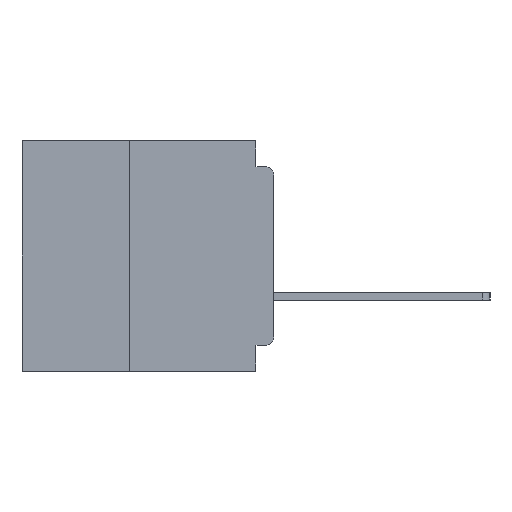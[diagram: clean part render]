
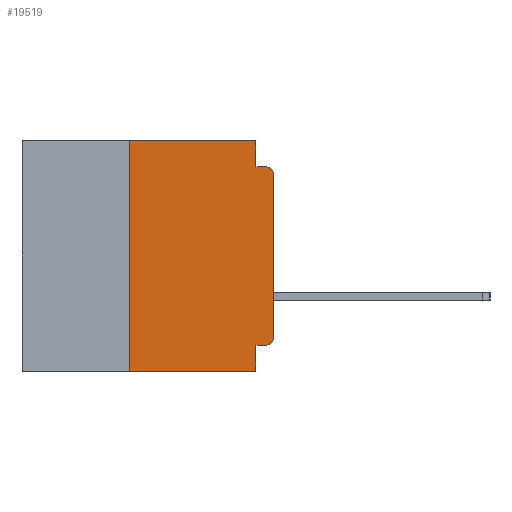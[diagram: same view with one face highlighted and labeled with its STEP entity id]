
A CAD part, left-side view. The second image highlights one B-rep face of the part: STEP entity #19519.
In plain terms, the highlighted planar face has unit normal (-1, 0, 0).
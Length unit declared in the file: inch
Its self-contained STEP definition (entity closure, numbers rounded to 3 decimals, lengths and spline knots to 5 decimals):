
#126 = ORIENTED_EDGE ( 'NONE', *, *, #12159, .T. ) ;
#327 = ORIENTED_EDGE ( 'NONE', *, *, #18618, .T. ) ;
#857 = ORIENTED_EDGE ( 'NONE', *, *, #13022, .F. ) ;
#1304 = ORIENTED_EDGE ( 'NONE', *, *, #26795, .F. ) ;
#1776 = LINE ( 'NONE', #21412, #37938 ) ;
#1802 = AXIS2_PLACEMENT_3D ( 'NONE', #40153, #40103, #40090 ) ;
#2200 = LINE ( 'NONE', #25122, #36204 ) ;
#2381 = CARTESIAN_POINT ( 'NONE',  ( 0., 0.25, -0.4 ) ) ;
#2428 = EDGE_CURVE ( 'NONE', #28921, #13755, #2200, .T. ) ;
#3907 = ORIENTED_EDGE ( 'NONE', *, *, #2428, .F. ) ;
#3928 = DIRECTION ( 'NONE',  ( 0., 0., 1. ) ) ;
#4588 = LINE ( 'NONE', #12384, #31452 ) ;
#4768 = CARTESIAN_POINT ( 'NONE',  ( 0., 0.437, 0. ) ) ;
#5545 = LINE ( 'NONE', #24265, #41652 ) ;
#5614 = VERTEX_POINT ( 'NONE', #10457 ) ;
#5684 = DIRECTION ( 'NONE',  ( 0., 1., 0. ) ) ;
#6616 = CARTESIAN_POINT ( 'NONE',  ( 0., 0.015, -0.045 ) ) ;
#6877 = EDGE_CURVE ( 'NONE', #5614, #39011, #18066, .T. ) ;
#7817 = ORIENTED_EDGE ( 'NONE', *, *, #22107, .F. ) ;
#8305 = DIRECTION ( 'NONE',  ( 0., 0., -1. ) ) ;
#8378 = ORIENTED_EDGE ( 'NONE', *, *, #15038, .T. ) ;
#8770 = CARTESIAN_POINT ( 'NONE',  ( 0., 0., -0.045 ) ) ;
#8804 = VECTOR ( 'NONE', #36818, 39.37008 ) ;
#10457 = CARTESIAN_POINT ( 'NONE',  ( 0., 0.015, -0.355 ) ) ;
#10784 = ORIENTED_EDGE ( 'NONE', *, *, #12684, .F. ) ;
#10994 = ORIENTED_EDGE ( 'NONE', *, *, #32732, .F. ) ;
#12159 = EDGE_CURVE ( 'NONE', #39011, #40071, #1776, .T. ) ;
#12169 = ORIENTED_EDGE ( 'NONE', *, *, #6877, .T. ) ;
#12384 = CARTESIAN_POINT ( 'NONE',  ( 0., 0.031, 0. ) ) ;
#12684 = EDGE_CURVE ( 'NONE', #27135, #31241, #5545, .T. ) ;
#13022 = EDGE_CURVE ( 'NONE', #45213, #23433, #44838, .T. ) ;
#13112 = CARTESIAN_POINT ( 'NONE',  ( 0., 0.437, -0.4 ) ) ;
#13446 = LINE ( 'NONE', #44415, #22800 ) ;
#13755 = VERTEX_POINT ( 'NONE', #16778 ) ;
#15038 = EDGE_CURVE ( 'NONE', #40482, #31241, #15154, .T. ) ;
#15154 = LINE ( 'NONE', #13112, #32748 ) ;
#16163 = EDGE_LOOP ( 'NONE', ( #126, #327, #857, #1304, #3907, #7817, #8378, #10784, #10994, #12169 ) ) ;
#16619 = DIRECTION ( 'NONE',  ( 0., -1., 0. ) ) ;
#16778 = CARTESIAN_POINT ( 'NONE',  ( 0., 0.031, 0. ) ) ;
#18066 = CIRCLE ( 'NONE', #1802, 0.015 ) ;
#18618 = EDGE_CURVE ( 'NONE', #40071, #23433, #29641, .T. ) ;
#19519 = ADVANCED_FACE ( 'NONE', ( #31757 ), #43129, .F. ) ;
#20160 = CARTESIAN_POINT ( 'NONE',  ( 0., 0.015, -0.06 ) ) ;
#21412 = CARTESIAN_POINT ( 'NONE',  ( 0., 0., 0. ) ) ;
#22107 = EDGE_CURVE ( 'NONE', #40482, #28921, #13446, .T. ) ;
#22800 = VECTOR ( 'NONE', #23560, 39.37008 ) ;
#23433 = VERTEX_POINT ( 'NONE', #6616 ) ;
#23560 = DIRECTION ( 'NONE',  ( 0., 0., 1. ) ) ;
#23681 = DIRECTION ( 'NONE',  ( 0., 0., -1. ) ) ;
#24265 = CARTESIAN_POINT ( 'NONE',  ( 0., 0.031, -0.4 ) ) ;
#24403 = DIRECTION ( 'NONE',  ( 0., 0., -1. ) ) ;
#24986 = DIRECTION ( 'NONE',  ( 0., -1., 0. ) ) ;
#25122 = CARTESIAN_POINT ( 'NONE',  ( 0., 0.437, 0. ) ) ;
#26795 = EDGE_CURVE ( 'NONE', #13755, #45213, #4588, .T. ) ;
#27135 = VERTEX_POINT ( 'NONE', #32001 ) ;
#27582 = AXIS2_PLACEMENT_3D ( 'NONE', #20160, #44542, #23681 ) ;
#27867 = CARTESIAN_POINT ( 'NONE',  ( 0., 0., -0.06 ) ) ;
#28921 = VERTEX_POINT ( 'NONE', #30355 ) ;
#29289 = DIRECTION ( 'NONE',  ( 1., 0., 0. ) ) ;
#29641 = CIRCLE ( 'NONE', #27582, 0.015 ) ;
#29874 = DIRECTION ( 'NONE',  ( 0., 0., -1. ) ) ;
#30204 = CARTESIAN_POINT ( 'NONE',  ( 0., 0., -0.355 ) ) ;
#30355 = CARTESIAN_POINT ( 'NONE',  ( 0., 0.25, 0. ) ) ;
#31241 = VERTEX_POINT ( 'NONE', #42178 ) ;
#31452 = VECTOR ( 'NONE', #29874, 39.37008 ) ;
#31757 = FACE_OUTER_BOUND ( 'NONE', #16163, .T. ) ;
#32001 = CARTESIAN_POINT ( 'NONE',  ( 0., 0.031, -0.355 ) ) ;
#32732 = EDGE_CURVE ( 'NONE', #5614, #27135, #43318, .T. ) ;
#32748 = VECTOR ( 'NONE', #16619, 39.37008 ) ;
#36204 = VECTOR ( 'NONE', #24986, 39.37008 ) ;
#36818 = DIRECTION ( 'NONE',  ( 0., -1., 0. ) ) ;
#37129 = CARTESIAN_POINT ( 'NONE',  ( 0., 0., -0.34 ) ) ;
#37938 = VECTOR ( 'NONE', #3928, 39.37008 ) ;
#39011 = VERTEX_POINT ( 'NONE', #37129 ) ;
#39851 = CARTESIAN_POINT ( 'NONE',  ( 0., 0.031, -0.045 ) ) ;
#40071 = VERTEX_POINT ( 'NONE', #27867 ) ;
#40090 = DIRECTION ( 'NONE',  ( 0., 0., -1. ) ) ;
#40103 = DIRECTION ( 'NONE',  ( -1., 0., 0. ) ) ;
#40153 = CARTESIAN_POINT ( 'NONE',  ( 0., 0.015, -0.34 ) ) ;
#40482 = VERTEX_POINT ( 'NONE', #2381 ) ;
#41345 = AXIS2_PLACEMENT_3D ( 'NONE', #4768, #29289, #8305 ) ;
#41652 = VECTOR ( 'NONE', #24403, 39.37008 ) ;
#42178 = CARTESIAN_POINT ( 'NONE',  ( 0., 0.031, -0.4 ) ) ;
#42234 = VECTOR ( 'NONE', #5684, 39.37008 ) ;
#43129 = PLANE ( 'NONE',  #41345 ) ;
#43318 = LINE ( 'NONE', #30204, #42234 ) ;
#44415 = CARTESIAN_POINT ( 'NONE',  ( 0., 0.25, -0.4 ) ) ;
#44542 = DIRECTION ( 'NONE',  ( -1., 0., 0. ) ) ;
#44838 = LINE ( 'NONE', #8770, #8804 ) ;
#45213 = VERTEX_POINT ( 'NONE', #39851 ) ;
